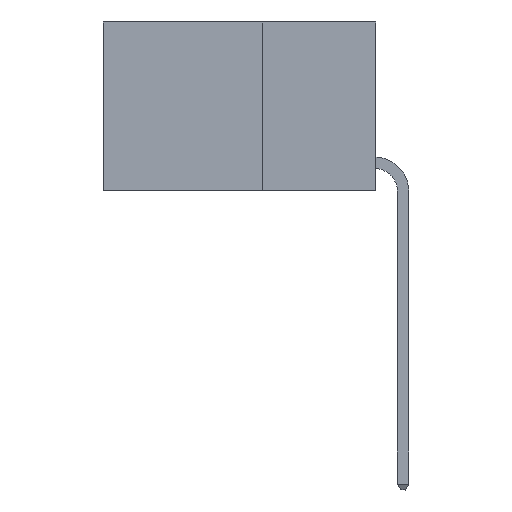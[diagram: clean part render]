
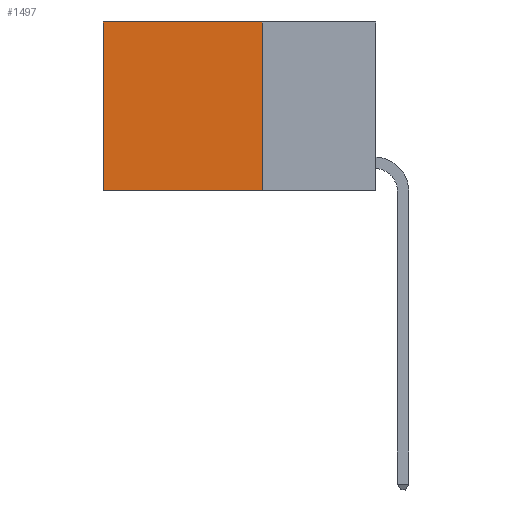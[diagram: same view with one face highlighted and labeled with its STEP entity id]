
A CAD part, left-side view. The second image highlights one B-rep face of the part: STEP entity #1497.
In plain terms, the highlighted planar face has unit normal (-1, 0, 0).
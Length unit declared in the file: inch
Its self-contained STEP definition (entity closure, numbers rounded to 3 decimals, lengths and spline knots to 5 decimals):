
#71 = CARTESIAN_POINT ( 'NONE',  ( 0.2625, 0.6, 0. ) ) ;
#262 = VERTEX_POINT ( 'NONE', #17782 ) ;
#1332 = VERTEX_POINT ( 'NONE', #20028 ) ;
#1497 = ADVANCED_FACE ( 'NONE', ( #15757 ), #23332, .F. ) ;
#2324 = CARTESIAN_POINT ( 'NONE',  ( 0.2625, 0.25, -0.37 ) ) ;
#3524 = CARTESIAN_POINT ( 'NONE',  ( 0.2625, 0.25, 0. ) ) ;
#5340 = LINE ( 'NONE', #71, #9939 ) ;
#5680 = EDGE_CURVE ( 'NONE', #10708, #23226, #11289, .T. ) ;
#6675 = ORIENTED_EDGE ( 'NONE', *, *, #10494, .T. ) ;
#6951 = LINE ( 'NONE', #3524, #11354 ) ;
#7615 = EDGE_CURVE ( 'NONE', #262, #10708, #12935, .T. ) ;
#8231 = ORIENTED_EDGE ( 'NONE', *, *, #14026, .T. ) ;
#8869 = CARTESIAN_POINT ( 'NONE',  ( 0.2625, 0.25, -0.37 ) ) ;
#9480 = DIRECTION ( 'NONE',  ( 0., 1., 0. ) ) ;
#9939 = VECTOR ( 'NONE', #13042, 39.37008 ) ;
#10494 = EDGE_CURVE ( 'NONE', #1332, #23226, #5340, .T. ) ;
#10708 = VERTEX_POINT ( 'NONE', #2324 ) ;
#11289 = LINE ( 'NONE', #8869, #15153 ) ;
#11354 = VECTOR ( 'NONE', #24057, 39.37008 ) ;
#12736 = AXIS2_PLACEMENT_3D ( 'NONE', #17341, #21134, #17460 ) ;
#12935 = LINE ( 'NONE', #20476, #14617 ) ;
#12949 = ORIENTED_EDGE ( 'NONE', *, *, #5680, .F. ) ;
#13042 = DIRECTION ( 'NONE',  ( 0., 0., -1. ) ) ;
#14026 = EDGE_CURVE ( 'NONE', #262, #1332, #6951, .T. ) ;
#14512 = ORIENTED_EDGE ( 'NONE', *, *, #7615, .F. ) ;
#14617 = VECTOR ( 'NONE', #20724, 39.37008 ) ;
#15153 = VECTOR ( 'NONE', #9480, 39.37008 ) ;
#15562 = CARTESIAN_POINT ( 'NONE',  ( 0.2625, 0.6, -0.37 ) ) ;
#15579 = EDGE_LOOP ( 'NONE', ( #6675, #12949, #14512, #8231 ) ) ;
#15757 = FACE_OUTER_BOUND ( 'NONE', #15579, .T. ) ;
#17341 = CARTESIAN_POINT ( 'NONE',  ( 0.2625, 0.25, 0. ) ) ;
#17460 = DIRECTION ( 'NONE',  ( 0., 0., -1. ) ) ;
#17782 = CARTESIAN_POINT ( 'NONE',  ( 0.2625, 0.25, 0. ) ) ;
#20028 = CARTESIAN_POINT ( 'NONE',  ( 0.2625, 0.6, 0. ) ) ;
#20476 = CARTESIAN_POINT ( 'NONE',  ( 0.2625, 0.25, 0. ) ) ;
#20724 = DIRECTION ( 'NONE',  ( 0., 0., -1. ) ) ;
#21134 = DIRECTION ( 'NONE',  ( 1., 0., 0. ) ) ;
#23226 = VERTEX_POINT ( 'NONE', #15562 ) ;
#23332 = PLANE ( 'NONE',  #12736 ) ;
#24057 = DIRECTION ( 'NONE',  ( 0., 1., 0. ) ) ;
